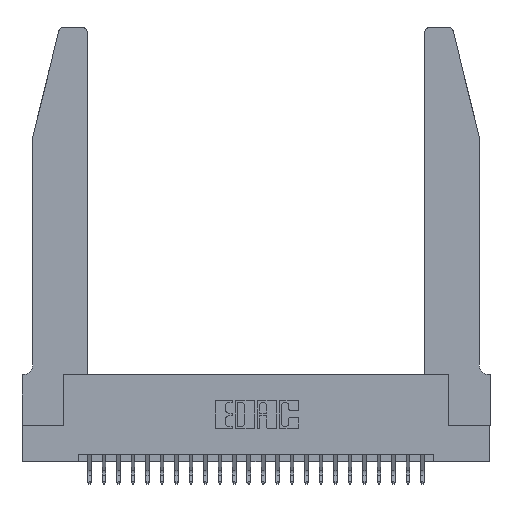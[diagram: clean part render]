
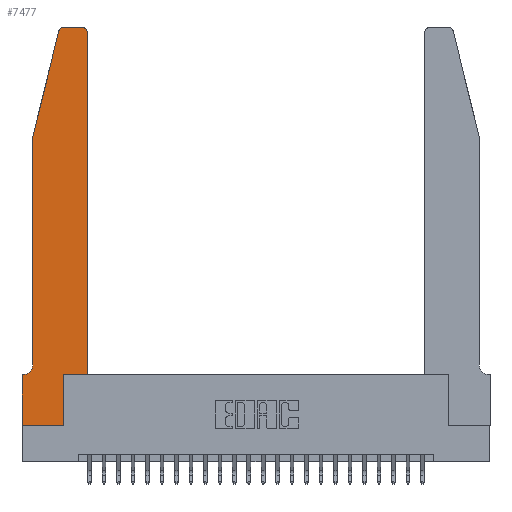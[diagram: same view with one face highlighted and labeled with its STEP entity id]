
A CAD part, top view. The second image highlights one B-rep face of the part: STEP entity #7477.
In plain terms, the highlighted planar face has unit normal (0, 0, 1).
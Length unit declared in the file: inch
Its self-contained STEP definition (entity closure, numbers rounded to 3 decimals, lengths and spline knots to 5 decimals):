
#253 = AXIS2_PLACEMENT_3D ( 'NONE', #3316, #19595, #5559 ) ;
#499 = CARTESIAN_POINT ( 'NONE',  ( 0.4505, 2.72, 0.37 ) ) ;
#687 = DIRECTION ( 'NONE',  ( 1., 0., 0. ) ) ;
#1593 = CARTESIAN_POINT ( 'NONE',  ( 0.2865, 0.35, 0.37 ) ) ;
#1645 = VECTOR ( 'NONE', #19587, 39.37008 ) ;
#1696 = EDGE_CURVE ( 'NONE', #15517, #11119, #21980, .T. ) ;
#1759 = ORIENTED_EDGE ( 'NONE', *, *, #3144, .T. ) ;
#1760 = ORIENTED_EDGE ( 'NONE', *, *, #7091, .T. ) ;
#1962 = DIRECTION ( 'NONE',  ( 0., 0., 1. ) ) ;
#2529 = DIRECTION ( 'NONE',  ( 0., 1., 0. ) ) ;
#2653 = EDGE_LOOP ( 'NONE', ( #9148, #24774, #6115, #8944, #17706, #24780, #10028, #3008, #12593, #1760, #1759, #16296 ) ) ;
#2764 = CARTESIAN_POINT ( 'NONE',  ( 0.2865, 0., 0.37 ) ) ;
#3008 = ORIENTED_EDGE ( 'NONE', *, *, #20964, .T. ) ;
#3144 = EDGE_CURVE ( 'NONE', #19101, #8631, #22902, .T. ) ;
#3316 = CARTESIAN_POINT ( 'NONE',  ( 0.284, 2.72, 0.37 ) ) ;
#3488 = EDGE_CURVE ( 'NONE', #19926, #23585, #23198, .T. ) ;
#3638 = AXIS2_PLACEMENT_3D ( 'NONE', #14048, #1962, #16206 ) ;
#4470 = CARTESIAN_POINT ( 'NONE',  ( 0.4205, 2.75, 0.37 ) ) ;
#4640 = CARTESIAN_POINT ( 'NONE',  ( 0., 0., 0.37 ) ) ;
#4720 = DIRECTION ( 'NONE',  ( 1., 0., 0. ) ) ;
#4998 = EDGE_CURVE ( 'NONE', #8631, #19006, #21466, .T. ) ;
#5008 = CARTESIAN_POINT ( 'NONE',  ( 0.4505, 0.35, 0.37 ) ) ;
#5494 = CARTESIAN_POINT ( 'NONE',  ( 0., 0.35, 0.37 ) ) ;
#5559 = DIRECTION ( 'NONE',  ( 1., 0., 0. ) ) ;
#5803 = CARTESIAN_POINT ( 'NONE',  ( 0.0055, 0.42, 0.37 ) ) ;
#6115 = ORIENTED_EDGE ( 'NONE', *, *, #23302, .T. ) ;
#6224 = EDGE_CURVE ( 'NONE', #19006, #18323, #7430, .T. ) ;
#6353 = CIRCLE ( 'NONE', #253, 0.03 ) ;
#6757 = VECTOR ( 'NONE', #23393, 39.37008 ) ;
#7091 = EDGE_CURVE ( 'NONE', #16422, #19101, #9886, .T. ) ;
#7430 = LINE ( 'NONE', #13559, #6757 ) ;
#7477 = ADVANCED_FACE ( 'NONE', ( #24773 ), #14578, .T. ) ;
#7507 = LINE ( 'NONE', #25096, #17681 ) ;
#7640 = AXIS2_PLACEMENT_3D ( 'NONE', #5494, #20199, #12437 ) ;
#7947 = EDGE_CURVE ( 'NONE', #18323, #10637, #6353, .T. ) ;
#8631 = VERTEX_POINT ( 'NONE', #499 ) ;
#8944 = ORIENTED_EDGE ( 'NONE', *, *, #17912, .T. ) ;
#9148 = ORIENTED_EDGE ( 'NONE', *, *, #6224, .T. ) ;
#9670 = CARTESIAN_POINT ( 'NONE',  ( 0.4505, 0.35, 0.37 ) ) ;
#9886 = LINE ( 'NONE', #9670, #13072 ) ;
#10028 = ORIENTED_EDGE ( 'NONE', *, *, #1696, .T. ) ;
#10210 = AXIS2_PLACEMENT_3D ( 'NONE', #5803, #20343, #12234 ) ;
#10376 = VECTOR ( 'NONE', #687, 39.37008 ) ;
#10637 = VERTEX_POINT ( 'NONE', #13336 ) ;
#11119 = VERTEX_POINT ( 'NONE', #12627 ) ;
#11273 = CARTESIAN_POINT ( 'NONE',  ( 0.0755, 2., 0.37 ) ) ;
#11558 = CARTESIAN_POINT ( 'NONE',  ( 0.0755, 2., 0.37 ) ) ;
#11616 = CARTESIAN_POINT ( 'NONE',  ( 0., 0., 0.37 ) ) ;
#11834 = VECTOR ( 'NONE', #15392, 39.37008 ) ;
#12234 = DIRECTION ( 'NONE',  ( -1., 0., 0. ) ) ;
#12437 = DIRECTION ( 'NONE',  ( 1., 0., 0. ) ) ;
#12593 = ORIENTED_EDGE ( 'NONE', *, *, #24594, .T. ) ;
#12627 = CARTESIAN_POINT ( 'NONE',  ( 0., 0., 0.37 ) ) ;
#13072 = VECTOR ( 'NONE', #4720, 39.37008 ) ;
#13336 = CARTESIAN_POINT ( 'NONE',  ( 0.25487, 2.72718, 0.37 ) ) ;
#13559 = CARTESIAN_POINT ( 'NONE',  ( 0.2605, 2.75, 0.37 ) ) ;
#13625 = DIRECTION ( 'NONE',  ( 0., -1., 0. ) ) ;
#14048 = CARTESIAN_POINT ( 'NONE',  ( 0.4205, 2.72, 0.37 ) ) ;
#14578 = PLANE ( 'NONE',  #7640 ) ;
#15061 = VERTEX_POINT ( 'NONE', #2764 ) ;
#15262 = DIRECTION ( 'NONE',  ( 0., 1., 0. ) ) ;
#15392 = DIRECTION ( 'NONE',  ( -0.239, -0.971, 0. ) ) ;
#15517 = VERTEX_POINT ( 'NONE', #22350 ) ;
#15586 = VECTOR ( 'NONE', #13625, 39.37008 ) ;
#16206 = DIRECTION ( 'NONE',  ( 1., 0., 0. ) ) ;
#16296 = ORIENTED_EDGE ( 'NONE', *, *, #4998, .T. ) ;
#16422 = VERTEX_POINT ( 'NONE', #1593 ) ;
#17681 = VECTOR ( 'NONE', #23433, 39.37008 ) ;
#17690 = EDGE_CURVE ( 'NONE', #23585, #15517, #7507, .T. ) ;
#17706 = ORIENTED_EDGE ( 'NONE', *, *, #3488, .T. ) ;
#17912 = EDGE_CURVE ( 'NONE', #19511, #19926, #20969, .T. ) ;
#17923 = CARTESIAN_POINT ( 'NONE',  ( 0.0755, 0.42, 0.37 ) ) ;
#18323 = VERTEX_POINT ( 'NONE', #23620 ) ;
#18468 = CARTESIAN_POINT ( 'NONE',  ( 0.0755, 2., 0.37 ) ) ;
#18667 = VECTOR ( 'NONE', #2529, 39.37008 ) ;
#19006 = VERTEX_POINT ( 'NONE', #4470 ) ;
#19101 = VERTEX_POINT ( 'NONE', #5008 ) ;
#19256 = CARTESIAN_POINT ( 'NONE',  ( 0.4505, 0.35, 0.37 ) ) ;
#19511 = VERTEX_POINT ( 'NONE', #18468 ) ;
#19587 = DIRECTION ( 'NONE',  ( 0., -1., 0. ) ) ;
#19595 = DIRECTION ( 'NONE',  ( 0., 0., 1. ) ) ;
#19926 = VERTEX_POINT ( 'NONE', #17923 ) ;
#20199 = DIRECTION ( 'NONE',  ( 0., 0., 1. ) ) ;
#20261 = LINE ( 'NONE', #20472, #18667 ) ;
#20343 = DIRECTION ( 'NONE',  ( 0., 0., -1. ) ) ;
#20472 = CARTESIAN_POINT ( 'NONE',  ( 0.2865, 0.35, 0.37 ) ) ;
#20760 = LINE ( 'NONE', #11273, #11834 ) ;
#20964 = EDGE_CURVE ( 'NONE', #11119, #15061, #22776, .T. ) ;
#20969 = LINE ( 'NONE', #11558, #15586 ) ;
#21466 = CIRCLE ( 'NONE', #3638, 0.03 ) ;
#21980 = LINE ( 'NONE', #11616, #1645 ) ;
#22350 = CARTESIAN_POINT ( 'NONE',  ( 0., 0.35, 0.37 ) ) ;
#22776 = LINE ( 'NONE', #4640, #10376 ) ;
#22902 = LINE ( 'NONE', #19256, #24757 ) ;
#23198 = CIRCLE ( 'NONE', #10210, 0.07 ) ;
#23302 = EDGE_CURVE ( 'NONE', #10637, #19511, #20760, .T. ) ;
#23393 = DIRECTION ( 'NONE',  ( -1., 0., 0. ) ) ;
#23433 = DIRECTION ( 'NONE',  ( -1., 0., 0. ) ) ;
#23585 = VERTEX_POINT ( 'NONE', #24176 ) ;
#23620 = CARTESIAN_POINT ( 'NONE',  ( 0.284, 2.75, 0.37 ) ) ;
#24176 = CARTESIAN_POINT ( 'NONE',  ( 0.0055, 0.35, 0.37 ) ) ;
#24594 = EDGE_CURVE ( 'NONE', #15061, #16422, #20261, .T. ) ;
#24757 = VECTOR ( 'NONE', #15262, 39.37008 ) ;
#24773 = FACE_OUTER_BOUND ( 'NONE', #2653, .T. ) ;
#24774 = ORIENTED_EDGE ( 'NONE', *, *, #7947, .T. ) ;
#24780 = ORIENTED_EDGE ( 'NONE', *, *, #17690, .T. ) ;
#25096 = CARTESIAN_POINT ( 'NONE',  ( 0.0755, 0.35, 0.37 ) ) ;
